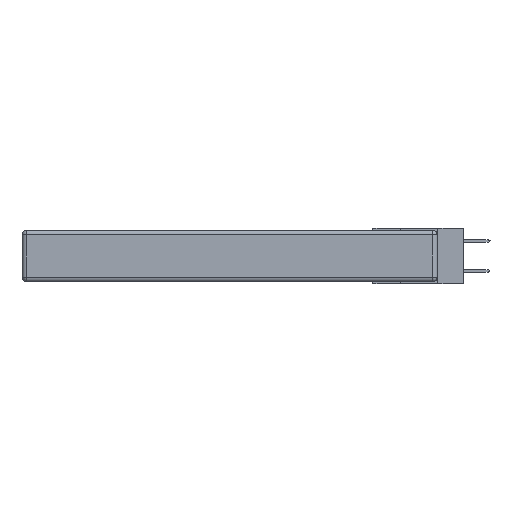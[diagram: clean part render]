
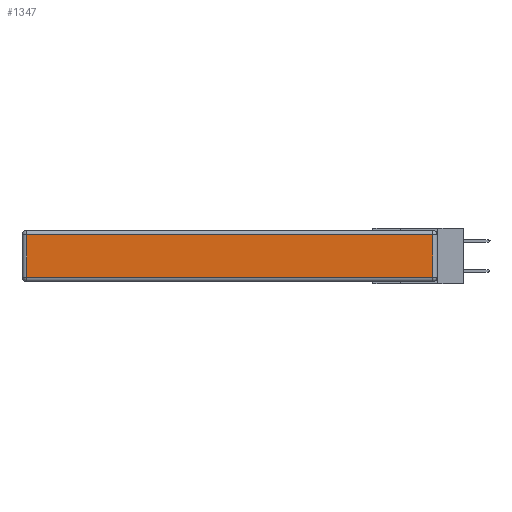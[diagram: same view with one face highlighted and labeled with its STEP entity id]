
A CAD part, left-side view. The second image highlights one B-rep face of the part: STEP entity #1347.
In plain terms, the highlighted planar face has unit normal (-1, 0, 0).
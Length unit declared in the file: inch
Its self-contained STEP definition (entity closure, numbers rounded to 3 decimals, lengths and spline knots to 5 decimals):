
#158 = VERTEX_POINT ( 'NONE', #4783 ) ;
#526 = ORIENTED_EDGE ( 'NONE', *, *, #10017, .T. ) ;
#1241 = DIRECTION ( 'NONE',  ( -1., 0., 0. ) ) ;
#1347 = ADVANCED_FACE ( 'NONE', ( #15389 ), #9124, .T. ) ;
#1356 = VECTOR ( 'NONE', #16007, 39.37008 ) ;
#1841 = EDGE_CURVE ( 'NONE', #6616, #10730, #16006, .T. ) ;
#2174 = CARTESIAN_POINT ( 'NONE',  ( 0., 2.75, -0.03 ) ) ;
#3713 = CARTESIAN_POINT ( 'NONE',  ( 0., 2.72, -0.343 ) ) ;
#3945 = CARTESIAN_POINT ( 'NONE',  ( 0., 2.72, -0.03 ) ) ;
#4726 = LINE ( 'NONE', #13296, #1356 ) ;
#4783 = CARTESIAN_POINT ( 'NONE',  ( 0., 0.03, -0.313 ) ) ;
#6197 = CARTESIAN_POINT ( 'NONE',  ( 0., 0., -0.313 ) ) ;
#6597 = DIRECTION ( 'NONE',  ( 0., 0., 1. ) ) ;
#6616 = VERTEX_POINT ( 'NONE', #3945 ) ;
#6930 = EDGE_CURVE ( 'NONE', #10730, #158, #12196, .T. ) ;
#7253 = EDGE_CURVE ( 'NONE', #7687, #6616, #15523, .T. ) ;
#7687 = VERTEX_POINT ( 'NONE', #16927 ) ;
#8604 = VECTOR ( 'NONE', #15630, 39.37008 ) ;
#8621 = VECTOR ( 'NONE', #15705, 39.37008 ) ;
#9124 = PLANE ( 'NONE',  #16814 ) ;
#10017 = EDGE_CURVE ( 'NONE', #158, #7687, #4726, .T. ) ;
#10730 = VERTEX_POINT ( 'NONE', #13953 ) ;
#11032 = ORIENTED_EDGE ( 'NONE', *, *, #1841, .T. ) ;
#11859 = ORIENTED_EDGE ( 'NONE', *, *, #7253, .T. ) ;
#11933 = CARTESIAN_POINT ( 'NONE',  ( 0., 0., -0.343 ) ) ;
#12196 = LINE ( 'NONE', #6197, #8604 ) ;
#13296 = CARTESIAN_POINT ( 'NONE',  ( 0., 0.03, -0.343 ) ) ;
#13463 = ORIENTED_EDGE ( 'NONE', *, *, #6930, .T. ) ;
#13953 = CARTESIAN_POINT ( 'NONE',  ( 0., 2.72, -0.313 ) ) ;
#15119 = VECTOR ( 'NONE', #17207, 39.37008 ) ;
#15389 = FACE_OUTER_BOUND ( 'NONE', #16893, .T. ) ;
#15523 = LINE ( 'NONE', #2174, #15119 ) ;
#15630 = DIRECTION ( 'NONE',  ( 0., -1., 0. ) ) ;
#15705 = DIRECTION ( 'NONE',  ( 0., 0., -1. ) ) ;
#16006 = LINE ( 'NONE', #3713, #8621 ) ;
#16007 = DIRECTION ( 'NONE',  ( 0., 0., 1. ) ) ;
#16814 = AXIS2_PLACEMENT_3D ( 'NONE', #11933, #1241, #6597 ) ;
#16893 = EDGE_LOOP ( 'NONE', ( #13463, #526, #11859, #11032 ) ) ;
#16927 = CARTESIAN_POINT ( 'NONE',  ( 0., 0.03, -0.03 ) ) ;
#17207 = DIRECTION ( 'NONE',  ( 0., 1., 0. ) ) ;
